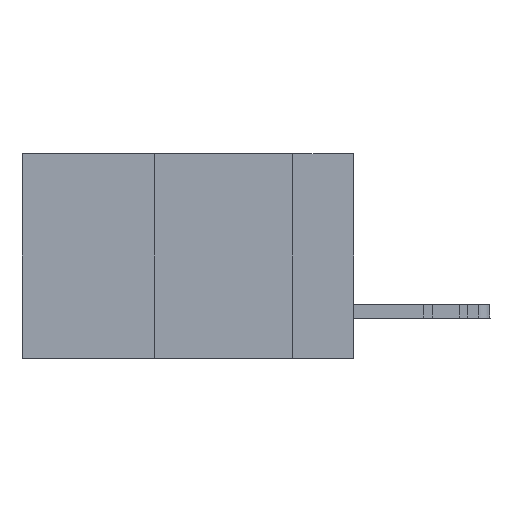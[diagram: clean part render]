
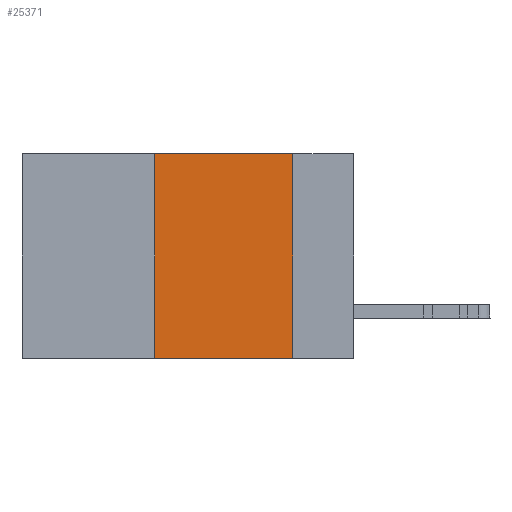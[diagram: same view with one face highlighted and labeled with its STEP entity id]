
A CAD part, left-side view. The second image highlights one B-rep face of the part: STEP entity #25371.
In plain terms, the highlighted planar face has unit normal (-1, 0, 0).
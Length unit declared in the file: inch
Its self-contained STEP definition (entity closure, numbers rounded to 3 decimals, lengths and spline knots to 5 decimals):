
#90 = LINE ( 'NONE', #3360, #32225 ) ;
#3360 = CARTESIAN_POINT ( 'NONE',  ( 0., 0.6, -0.37 ) ) ;
#4187 = CARTESIAN_POINT ( 'NONE',  ( 0., 0.6, 0. ) ) ;
#5256 = VECTOR ( 'NONE', #48575, 39.37008 ) ;
#8080 = PLANE ( 'NONE',  #46531 ) ;
#10389 = VERTEX_POINT ( 'NONE', #44290 ) ;
#13766 = LINE ( 'NONE', #49394, #22235 ) ;
#14526 = DIRECTION ( 'NONE',  ( 0., 0., 1. ) ) ;
#14666 = EDGE_LOOP ( 'NONE', ( #34521, #48964, #17556, #15301 ) ) ;
#15301 = ORIENTED_EDGE ( 'NONE', *, *, #40851, .T. ) ;
#15852 = VERTEX_POINT ( 'NONE', #16378 ) ;
#16378 = CARTESIAN_POINT ( 'NONE',  ( 0., 0.36, -0.37 ) ) ;
#17556 = ORIENTED_EDGE ( 'NONE', *, *, #32973, .F. ) ;
#21667 = LINE ( 'NONE', #44514, #5256 ) ;
#22235 = VECTOR ( 'NONE', #14526, 39.37008 ) ;
#22531 = DIRECTION ( 'NONE',  ( 0., -1., 0. ) ) ;
#23918 = EDGE_CURVE ( 'NONE', #10389, #37389, #40835, .T. ) ;
#25371 = ADVANCED_FACE ( 'NONE', ( #26126 ), #8080, .F. ) ;
#26126 = FACE_OUTER_BOUND ( 'NONE', #14666, .T. ) ;
#27061 = EDGE_CURVE ( 'NONE', #34085, #10389, #21667, .T. ) ;
#30115 = CARTESIAN_POINT ( 'NONE',  ( 0., 0.11, 0. ) ) ;
#30430 = DIRECTION ( 'NONE',  ( 0., 0., -1. ) ) ;
#31604 = DIRECTION ( 'NONE',  ( 1., 0., 0. ) ) ;
#32225 = VECTOR ( 'NONE', #22531, 39.37008 ) ;
#32973 = EDGE_CURVE ( 'NONE', #15852, #34085, #13766, .T. ) ;
#34085 = VERTEX_POINT ( 'NONE', #41172 ) ;
#34521 = ORIENTED_EDGE ( 'NONE', *, *, #23918, .F. ) ;
#35184 = DIRECTION ( 'NONE',  ( 0., 0., -1. ) ) ;
#35964 = CARTESIAN_POINT ( 'NONE',  ( 0., 0.11, -0.37 ) ) ;
#37389 = VERTEX_POINT ( 'NONE', #35964 ) ;
#39604 = VECTOR ( 'NONE', #30430, 39.37008 ) ;
#40835 = LINE ( 'NONE', #30115, #39604 ) ;
#40851 = EDGE_CURVE ( 'NONE', #15852, #37389, #90, .T. ) ;
#41172 = CARTESIAN_POINT ( 'NONE',  ( 0., 0.36, 0. ) ) ;
#44290 = CARTESIAN_POINT ( 'NONE',  ( 0., 0.11, 0. ) ) ;
#44514 = CARTESIAN_POINT ( 'NONE',  ( 0., 0.6, 0. ) ) ;
#46531 = AXIS2_PLACEMENT_3D ( 'NONE', #4187, #31604, #35184 ) ;
#48575 = DIRECTION ( 'NONE',  ( 0., -1., 0. ) ) ;
#48964 = ORIENTED_EDGE ( 'NONE', *, *, #27061, .F. ) ;
#49394 = CARTESIAN_POINT ( 'NONE',  ( 0., 0.36, 0. ) ) ;
